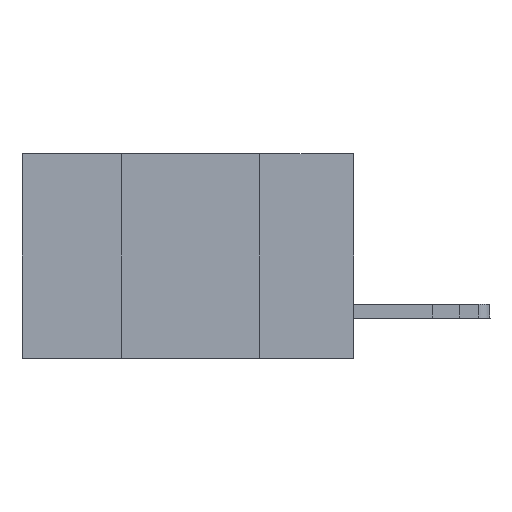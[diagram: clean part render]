
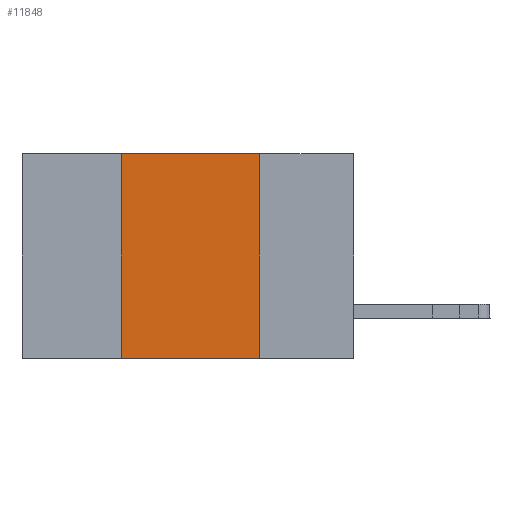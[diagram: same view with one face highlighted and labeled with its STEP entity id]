
A CAD part, left-side view. The second image highlights one B-rep face of the part: STEP entity #11848.
In plain terms, the highlighted planar face has unit normal (-1, 0, 0).
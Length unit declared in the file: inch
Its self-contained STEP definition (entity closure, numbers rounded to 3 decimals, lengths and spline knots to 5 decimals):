
#1000 = ORIENTED_EDGE ( 'NONE', *, *, #23999, .F. ) ;
#1147 = CARTESIAN_POINT ( 'NONE',  ( 0., 0.42, 0. ) ) ;
#1656 = DIRECTION ( 'NONE',  ( 0., 0., -1. ) ) ;
#1679 = CARTESIAN_POINT ( 'NONE',  ( 0., 0.17, -0.37 ) ) ;
#2506 = EDGE_CURVE ( 'NONE', #11687, #2576, #17489, .T. ) ;
#2576 = VERTEX_POINT ( 'NONE', #1679 ) ;
#3437 = VECTOR ( 'NONE', #10026, 39.37008 ) ;
#4657 = DIRECTION ( 'NONE',  ( 0., -1., 0. ) ) ;
#5930 = CARTESIAN_POINT ( 'NONE',  ( 0., 0.42, 0. ) ) ;
#6235 = EDGE_LOOP ( 'NONE', ( #23440, #11809, #1000, #8675 ) ) ;
#6671 = VECTOR ( 'NONE', #21846, 39.37008 ) ;
#6816 = CARTESIAN_POINT ( 'NONE',  ( 0., 0.17, 0. ) ) ;
#7534 = DIRECTION ( 'NONE',  ( 1., 0., 0. ) ) ;
#7902 = CARTESIAN_POINT ( 'NONE',  ( 0., 0.42, -0.37 ) ) ;
#8546 = EDGE_CURVE ( 'NONE', #16518, #2576, #15861, .T. ) ;
#8675 = ORIENTED_EDGE ( 'NONE', *, *, #8546, .T. ) ;
#9569 = DIRECTION ( 'NONE',  ( 0., 0., 1. ) ) ;
#10026 = DIRECTION ( 'NONE',  ( 0., -1., 0. ) ) ;
#11687 = VERTEX_POINT ( 'NONE', #22486 ) ;
#11809 = ORIENTED_EDGE ( 'NONE', *, *, #15718, .F. ) ;
#11848 = ADVANCED_FACE ( 'NONE', ( #17780 ), #13474, .F. ) ;
#13474 = PLANE ( 'NONE',  #21844 ) ;
#13769 = VERTEX_POINT ( 'NONE', #1147 ) ;
#14870 = LINE ( 'NONE', #17880, #3437 ) ;
#15408 = CARTESIAN_POINT ( 'NONE',  ( 0., 0.6, 0. ) ) ;
#15718 = EDGE_CURVE ( 'NONE', #13769, #11687, #14870, .T. ) ;
#15861 = LINE ( 'NONE', #23718, #20374 ) ;
#16518 = VERTEX_POINT ( 'NONE', #7902 ) ;
#17489 = LINE ( 'NONE', #6816, #6671 ) ;
#17780 = FACE_OUTER_BOUND ( 'NONE', #6235, .T. ) ;
#17880 = CARTESIAN_POINT ( 'NONE',  ( 0., 0.6, 0. ) ) ;
#18301 = VECTOR ( 'NONE', #9569, 39.37008 ) ;
#19497 = LINE ( 'NONE', #5930, #18301 ) ;
#20374 = VECTOR ( 'NONE', #4657, 39.37008 ) ;
#21844 = AXIS2_PLACEMENT_3D ( 'NONE', #15408, #7534, #1656 ) ;
#21846 = DIRECTION ( 'NONE',  ( 0., 0., -1. ) ) ;
#22486 = CARTESIAN_POINT ( 'NONE',  ( 0., 0.17, 0. ) ) ;
#23440 = ORIENTED_EDGE ( 'NONE', *, *, #2506, .F. ) ;
#23718 = CARTESIAN_POINT ( 'NONE',  ( 0., 0.6, -0.37 ) ) ;
#23999 = EDGE_CURVE ( 'NONE', #16518, #13769, #19497, .T. ) ;
